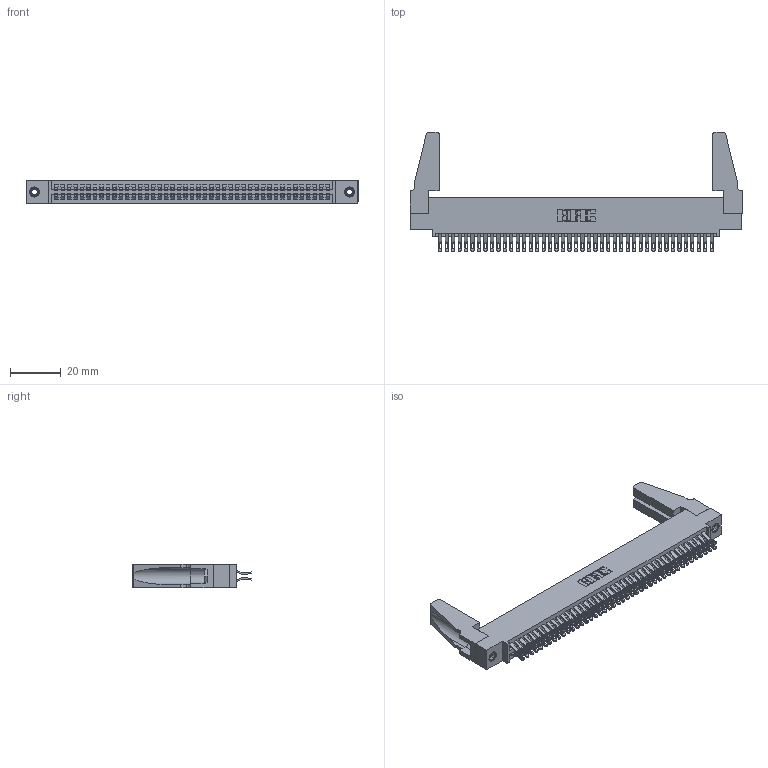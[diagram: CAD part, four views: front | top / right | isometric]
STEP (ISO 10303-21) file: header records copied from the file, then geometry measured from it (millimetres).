
FILE_DESCRIPTION (( 'STEP AP203' ), '1' );
FILE_NAME ('395-086-555-588.STEP', '2019-10-25T12:19:43', ( '' ), ( '' ), 'SwSTEP 2.0', 'SolidWorks 2016', '' );
FILE_SCHEMA (( 'CONFIG_CONTROL_DESIGN' ));
Length unit declared in the file: inch
Products named in the file (5): 345 Part_0.110 Offset - 0.156 Dia-TH; 345-292-001_555 Tail; 345-250-001_345-250-001-102; 345-220-078_345-220-088; 395-086-555-588
Assembly tree (91 placements, depth 2):
  395-086-555-588
    345 Part_0.110 Offset - 0.156 Dia-TH
    345-292-001_555 Tail  x86
    345-250-001_345-250-001-102  x2
    345-220-078_345-220-088  x2
Bounding box: 130.45 x 46.79 x 9.4 mm (x, y, z)
Volume: 16110.3 mm3; surface area: 23108 mm2
Topology: 91 solids, 91 shells, 5070 faces, 15889 edges, 10582 vertices
Faces by surface type: plane 2822, cylinder 2232, cone 12, torus 4
Entity records: 36210 total; most frequent: CARTESIAN_POINT 6100, ORIENTED_EDGE 5964, DIRECTION 5350, EDGE_CURVE 2982, VECTOR 2616, LINE 2616, VERTEX_POINT 1982, AXIS2_PLACEMENT_3D 1367
